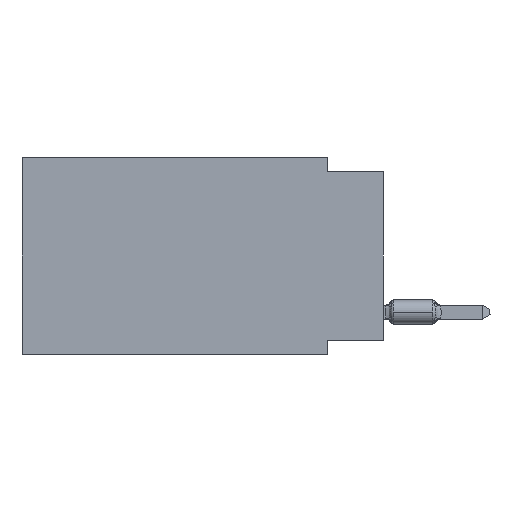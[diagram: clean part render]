
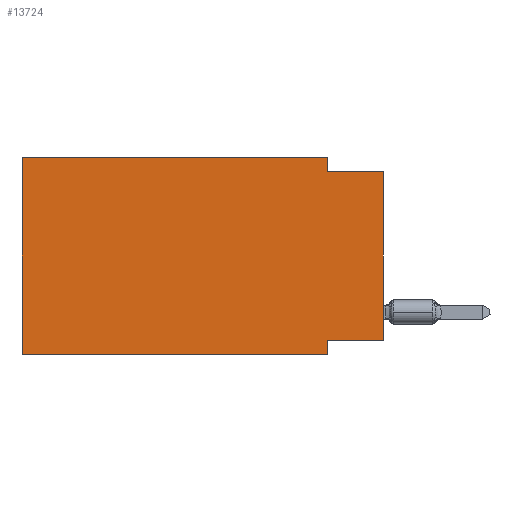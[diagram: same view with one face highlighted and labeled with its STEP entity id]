
A CAD part, left-side view. The second image highlights one B-rep face of the part: STEP entity #13724.
In plain terms, the highlighted planar face has unit normal (-1, 0, 0).
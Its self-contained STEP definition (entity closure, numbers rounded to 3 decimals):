
#910 = LINE ( 'NONE', #48988, #34227 ) ;
#1083 = EDGE_LOOP ( 'NONE', ( #53695, #18046, #9767, #10065, #43861, #46331, #36055, #31376 ) ) ;
#2029 = LINE ( 'NONE', #23125, #40950 ) ;
#2730 = CARTESIAN_POINT ( 'NONE',  ( 0., 2.54, -8.89 ) ) ;
#6717 = CARTESIAN_POINT ( 'NONE',  ( 0., 16.383, -8.89 ) ) ;
#7124 = VERTEX_POINT ( 'NONE', #36531 ) ;
#7682 = EDGE_CURVE ( 'NONE', #33483, #41971, #30070, .T. ) ;
#8417 = CARTESIAN_POINT ( 'NONE',  ( 0., 0., -8.255 ) ) ;
#8593 = CARTESIAN_POINT ( 'NONE',  ( 0., 0., -0.635 ) ) ;
#9767 = ORIENTED_EDGE ( 'NONE', *, *, #29079, .F. ) ;
#10065 = ORIENTED_EDGE ( 'NONE', *, *, #44925, .F. ) ;
#10279 = VERTEX_POINT ( 'NONE', #48435 ) ;
#11588 = CARTESIAN_POINT ( 'NONE',  ( 0., 2.54, 0. ) ) ;
#11593 = DIRECTION ( 'NONE',  ( 0., -1., 0. ) ) ;
#12121 = CARTESIAN_POINT ( 'NONE',  ( 0., 16.383, -8.89 ) ) ;
#13724 = ADVANCED_FACE ( 'NONE', ( #31329 ), #27482, .F. ) ;
#15177 = AXIS2_PLACEMENT_3D ( 'NONE', #23607, #48055, #39567 ) ;
#16003 = VERTEX_POINT ( 'NONE', #8593 ) ;
#16382 = VECTOR ( 'NONE', #48686, 1000. ) ;
#16604 = CARTESIAN_POINT ( 'NONE',  ( 0., 2.54, -0.635 ) ) ;
#16802 = VECTOR ( 'NONE', #11593, 1000. ) ;
#18046 = ORIENTED_EDGE ( 'NONE', *, *, #31521, .F. ) ;
#19338 = VECTOR ( 'NONE', #38579, 1000. ) ;
#19379 = CARTESIAN_POINT ( 'NONE',  ( 0., 0., -8.255 ) ) ;
#21559 = CARTESIAN_POINT ( 'NONE',  ( 0., 16.383, 0. ) ) ;
#21895 = EDGE_CURVE ( 'NONE', #36376, #7124, #31964, .T. ) ;
#22133 = EDGE_CURVE ( 'NONE', #33483, #16003, #2029, .T. ) ;
#23125 = CARTESIAN_POINT ( 'NONE',  ( 0., 0., 0. ) ) ;
#23607 = CARTESIAN_POINT ( 'NONE',  ( 0., 16.383, 0. ) ) ;
#24482 = DIRECTION ( 'NONE',  ( 0., 0., -1. ) ) ;
#25686 = EDGE_CURVE ( 'NONE', #36376, #51850, #50008, .T. ) ;
#27482 = PLANE ( 'NONE',  #15177 ) ;
#27530 = LINE ( 'NONE', #11588, #40581 ) ;
#29067 = CARTESIAN_POINT ( 'NONE',  ( 0., 2.54, -8.89 ) ) ;
#29079 = EDGE_CURVE ( 'NONE', #10279, #31736, #27530, .T. ) ;
#30070 = LINE ( 'NONE', #8417, #40091 ) ;
#31329 = FACE_OUTER_BOUND ( 'NONE', #1083, .T. ) ;
#31376 = ORIENTED_EDGE ( 'NONE', *, *, #7682, .F. ) ;
#31521 = EDGE_CURVE ( 'NONE', #31736, #16003, #910, .T. ) ;
#31736 = VERTEX_POINT ( 'NONE', #16604 ) ;
#31964 = LINE ( 'NONE', #45688, #16382 ) ;
#32891 = DIRECTION ( 'NONE',  ( 0., 0., -1. ) ) ;
#33483 = VERTEX_POINT ( 'NONE', #19379 ) ;
#34227 = VECTOR ( 'NONE', #45187, 1000. ) ;
#34342 = EDGE_CURVE ( 'NONE', #41971, #51850, #40590, .T. ) ;
#36055 = ORIENTED_EDGE ( 'NONE', *, *, #34342, .F. ) ;
#36376 = VERTEX_POINT ( 'NONE', #6717 ) ;
#36531 = CARTESIAN_POINT ( 'NONE',  ( 0., 16.383, 0. ) ) ;
#37844 = VECTOR ( 'NONE', #32891, 1000. ) ;
#38579 = DIRECTION ( 'NONE',  ( 0., -1., 0. ) ) ;
#39036 = DIRECTION ( 'NONE',  ( 0., 0., 1. ) ) ;
#39567 = DIRECTION ( 'NONE',  ( 0., 0., -1. ) ) ;
#40091 = VECTOR ( 'NONE', #46814, 1000. ) ;
#40581 = VECTOR ( 'NONE', #24482, 1000. ) ;
#40590 = LINE ( 'NONE', #2730, #37844 ) ;
#40950 = VECTOR ( 'NONE', #39036, 1000. ) ;
#41971 = VERTEX_POINT ( 'NONE', #45470 ) ;
#42695 = LINE ( 'NONE', #21559, #19338 ) ;
#43861 = ORIENTED_EDGE ( 'NONE', *, *, #21895, .F. ) ;
#44925 = EDGE_CURVE ( 'NONE', #7124, #10279, #42695, .T. ) ;
#45187 = DIRECTION ( 'NONE',  ( 0., -1., 0. ) ) ;
#45470 = CARTESIAN_POINT ( 'NONE',  ( 0., 2.54, -8.255 ) ) ;
#45688 = CARTESIAN_POINT ( 'NONE',  ( 0., 16.383, 0. ) ) ;
#46331 = ORIENTED_EDGE ( 'NONE', *, *, #25686, .T. ) ;
#46814 = DIRECTION ( 'NONE',  ( 0., 1., 0. ) ) ;
#48055 = DIRECTION ( 'NONE',  ( 1., 0., 0. ) ) ;
#48435 = CARTESIAN_POINT ( 'NONE',  ( 0., 2.54, 0. ) ) ;
#48686 = DIRECTION ( 'NONE',  ( 0., 0., 1. ) ) ;
#48988 = CARTESIAN_POINT ( 'NONE',  ( 0., 0., -0.635 ) ) ;
#50008 = LINE ( 'NONE', #12121, #16802 ) ;
#51850 = VERTEX_POINT ( 'NONE', #29067 ) ;
#53695 = ORIENTED_EDGE ( 'NONE', *, *, #22133, .T. ) ;
